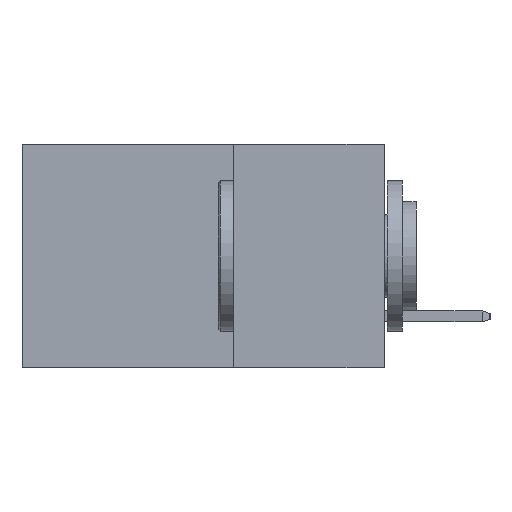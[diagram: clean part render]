
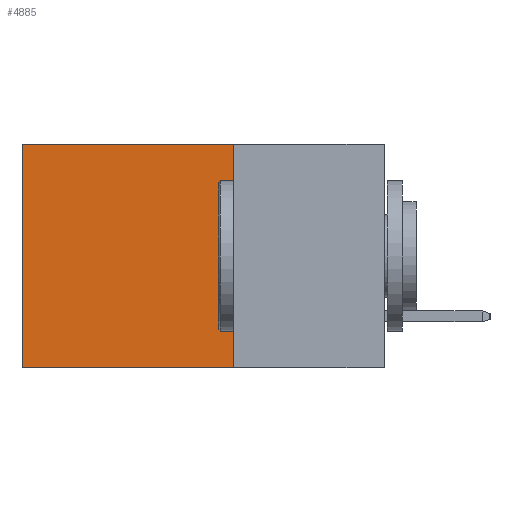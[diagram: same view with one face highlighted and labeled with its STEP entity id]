
A CAD part, left-side view. The second image highlights one B-rep face of the part: STEP entity #4885.
In plain terms, the highlighted planar face has unit normal (-1, 0, 0).
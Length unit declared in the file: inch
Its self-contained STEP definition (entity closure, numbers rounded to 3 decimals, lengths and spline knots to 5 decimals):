
#53 = PLANE ( 'NONE',  #4730 ) ;
#520 = DIRECTION ( 'NONE',  ( 0., 0., -1. ) ) ;
#532 = CARTESIAN_POINT ( 'NONE',  ( 0.2615, 0.25, 0. ) ) ;
#659 = DIRECTION ( 'NONE',  ( 1., 0., 0. ) ) ;
#1028 = DIRECTION ( 'NONE',  ( 0., 1., 0. ) ) ;
#1267 = EDGE_CURVE ( 'NONE', #16815, #19163, #17285, .T. ) ;
#3578 = CARTESIAN_POINT ( 'NONE',  ( 0.2615, 0.25, -0.37 ) ) ;
#3603 = DIRECTION ( 'NONE',  ( 0., 1., 0. ) ) ;
#4223 = ORIENTED_EDGE ( 'NONE', *, *, #5333, .T. ) ;
#4706 = EDGE_CURVE ( 'NONE', #19163, #14540, #7445, .T. ) ;
#4730 = AXIS2_PLACEMENT_3D ( 'NONE', #19346, #659, #520 ) ;
#4885 = ADVANCED_FACE ( 'NONE', ( #8245 ), #53, .F. ) ;
#5333 = EDGE_CURVE ( 'NONE', #16815, #8532, #22540, .T. ) ;
#6831 = ORIENTED_EDGE ( 'NONE', *, *, #11235, .T. ) ;
#7445 = LINE ( 'NONE', #3578, #16234 ) ;
#8032 = LINE ( 'NONE', #19633, #15726 ) ;
#8057 = DIRECTION ( 'NONE',  ( 0., 0., -1. ) ) ;
#8245 = FACE_OUTER_BOUND ( 'NONE', #20605, .T. ) ;
#8445 = CARTESIAN_POINT ( 'NONE',  ( 0.2615, 0.6, 0. ) ) ;
#8532 = VERTEX_POINT ( 'NONE', #8445 ) ;
#9933 = CARTESIAN_POINT ( 'NONE',  ( 0.2615, 0.25, 0. ) ) ;
#11235 = EDGE_CURVE ( 'NONE', #8532, #14540, #8032, .T. ) ;
#11478 = CARTESIAN_POINT ( 'NONE',  ( 0.2615, 0.25, -0.37 ) ) ;
#12067 = ORIENTED_EDGE ( 'NONE', *, *, #4706, .F. ) ;
#12615 = VECTOR ( 'NONE', #8057, 39.37008 ) ;
#13456 = VECTOR ( 'NONE', #1028, 39.37008 ) ;
#14188 = CARTESIAN_POINT ( 'NONE',  ( 0.2615, 0.6, -0.37 ) ) ;
#14540 = VERTEX_POINT ( 'NONE', #14188 ) ;
#15726 = VECTOR ( 'NONE', #20155, 39.37008 ) ;
#16234 = VECTOR ( 'NONE', #3603, 39.37008 ) ;
#16815 = VERTEX_POINT ( 'NONE', #9933 ) ;
#17285 = LINE ( 'NONE', #17669, #12615 ) ;
#17669 = CARTESIAN_POINT ( 'NONE',  ( 0.2615, 0.25, -0.37 ) ) ;
#19163 = VERTEX_POINT ( 'NONE', #11478 ) ;
#19346 = CARTESIAN_POINT ( 'NONE',  ( 0.2615, 0.25, -0.37 ) ) ;
#19633 = CARTESIAN_POINT ( 'NONE',  ( 0.2615, 0.6, -0.37 ) ) ;
#20155 = DIRECTION ( 'NONE',  ( 0., 0., -1. ) ) ;
#20605 = EDGE_LOOP ( 'NONE', ( #6831, #12067, #21911, #4223 ) ) ;
#21911 = ORIENTED_EDGE ( 'NONE', *, *, #1267, .F. ) ;
#22540 = LINE ( 'NONE', #532, #13456 ) ;
